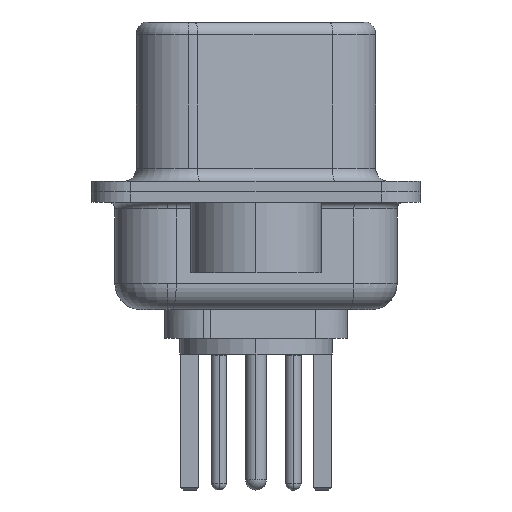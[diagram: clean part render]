
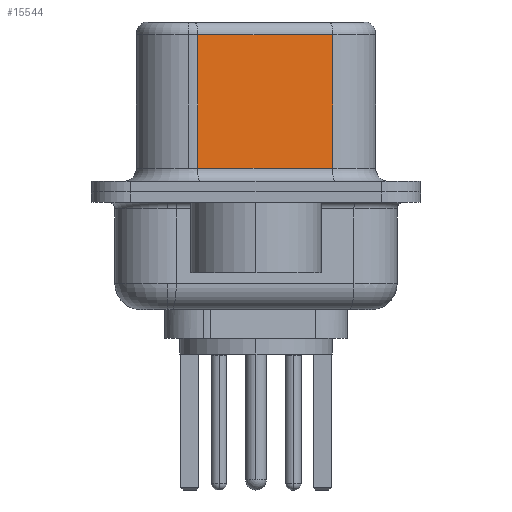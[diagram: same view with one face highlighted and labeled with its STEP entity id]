
A CAD part, left-side view. The second image highlights one B-rep face of the part: STEP entity #15544.
In plain terms, the highlighted planar face has unit normal (-0.985, -0.174, 0).
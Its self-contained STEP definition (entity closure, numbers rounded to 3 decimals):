
#229 = VERTEX_POINT ( 'NONE', #17821 ) ;
#616 = VECTOR ( 'NONE', #11098, 1000. ) ;
#3195 = PLANE ( 'NONE',  #6522 ) ;
#3250 = ORIENTED_EDGE ( 'NONE', *, *, #10139, .T. ) ;
#4005 = CARTESIAN_POINT ( 'NONE',  ( 4.585, -2.927, 6.02 ) ) ;
#4419 = LINE ( 'NONE', #16527, #17130 ) ;
#4880 = EDGE_CURVE ( 'NONE', #16808, #21624, #15049, .T. ) ;
#5806 = VECTOR ( 'NONE', #6512, 1000. ) ;
#6436 = DIRECTION ( 'NONE',  ( 0., 0., -1. ) ) ;
#6512 = DIRECTION ( 'NONE',  ( 0.174, -0.985, 0. ) ) ;
#6522 = AXIS2_PLACEMENT_3D ( 'NONE', #13361, #11893, #11681 ) ;
#7949 = EDGE_LOOP ( 'NONE', ( #16503, #3250, #11780, #14002 ) ) ;
#8068 = CARTESIAN_POINT ( 'NONE',  ( 3.675, 2.233, 6.02 ) ) ;
#9806 = CARTESIAN_POINT ( 'NONE',  ( 3.675, 2.233, 0.9 ) ) ;
#9917 = CARTESIAN_POINT ( 'NONE',  ( 3.675, 2.233, 6.52 ) ) ;
#10035 = LINE ( 'NONE', #18174, #5806 ) ;
#10139 = EDGE_CURVE ( 'NONE', #21907, #16808, #4419, .T. ) ;
#11098 = DIRECTION ( 'NONE',  ( 0., 0., -1. ) ) ;
#11450 = DIRECTION ( 'NONE',  ( -0.174, 0.985, 0. ) ) ;
#11681 = DIRECTION ( 'NONE',  ( -0.174, 0.985, 0. ) ) ;
#11692 = FACE_OUTER_BOUND ( 'NONE', #7949, .T. ) ;
#11780 = ORIENTED_EDGE ( 'NONE', *, *, #4880, .T. ) ;
#11893 = DIRECTION ( 'NONE',  ( 0.985, 0.174, 0. ) ) ;
#12898 = VECTOR ( 'NONE', #6436, 1000. ) ;
#13361 = CARTESIAN_POINT ( 'NONE',  ( 4.585, -2.927, 6.52 ) ) ;
#13382 = LINE ( 'NONE', #21465, #616 ) ;
#14002 = ORIENTED_EDGE ( 'NONE', *, *, #17560, .T. ) ;
#15049 = LINE ( 'NONE', #9917, #12898 ) ;
#15544 = ADVANCED_FACE ( 'NONE', ( #11692 ), #3195, .F. ) ;
#16503 = ORIENTED_EDGE ( 'NONE', *, *, #19930, .F. ) ;
#16527 = CARTESIAN_POINT ( 'NONE',  ( 4.585, -2.927, 6.02 ) ) ;
#16808 = VERTEX_POINT ( 'NONE', #8068 ) ;
#17130 = VECTOR ( 'NONE', #11450, 1000. ) ;
#17560 = EDGE_CURVE ( 'NONE', #21624, #229, #10035, .T. ) ;
#17821 = CARTESIAN_POINT ( 'NONE',  ( 4.585, -2.927, 0.9 ) ) ;
#18174 = CARTESIAN_POINT ( 'NONE',  ( 4.585, -2.927, 0.9 ) ) ;
#19930 = EDGE_CURVE ( 'NONE', #21907, #229, #13382, .T. ) ;
#21465 = CARTESIAN_POINT ( 'NONE',  ( 4.585, -2.927, 6.52 ) ) ;
#21624 = VERTEX_POINT ( 'NONE', #9806 ) ;
#21907 = VERTEX_POINT ( 'NONE', #4005 ) ;
